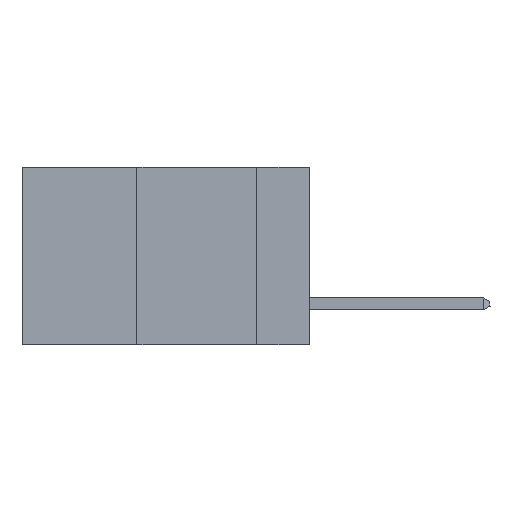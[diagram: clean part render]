
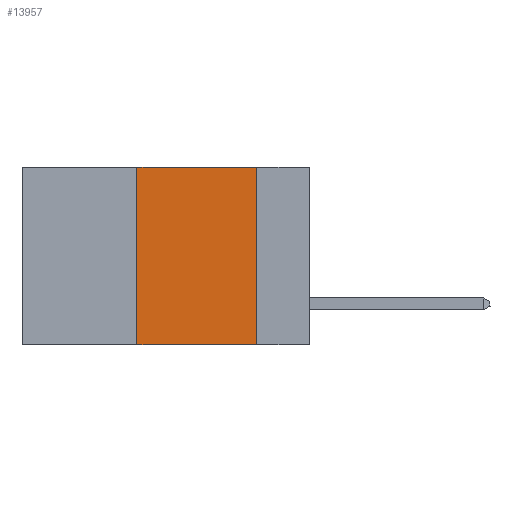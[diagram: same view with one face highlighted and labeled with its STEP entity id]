
A CAD part, left-side view. The second image highlights one B-rep face of the part: STEP entity #13957.
In plain terms, the highlighted planar face has unit normal (-1, 0, 0).
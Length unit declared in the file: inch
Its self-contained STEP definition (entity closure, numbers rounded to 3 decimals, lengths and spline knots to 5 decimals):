
#29 = CARTESIAN_POINT ( 'NONE',  ( 0., 0.6, 0. ) ) ;
#192 = EDGE_CURVE ( 'NONE', #10372, #8688, #6250, .T. ) ;
#811 = CARTESIAN_POINT ( 'NONE',  ( 0., 0.11, 0. ) ) ;
#1330 = DIRECTION ( 'NONE',  ( 0., -1., 0. ) ) ;
#1758 = DIRECTION ( 'NONE',  ( 0., 0., -1. ) ) ;
#2094 = VERTEX_POINT ( 'NONE', #15058 ) ;
#2177 = VECTOR ( 'NONE', #12289, 39.37008 ) ;
#3598 = EDGE_CURVE ( 'NONE', #16741, #2094, #14230, .T. ) ;
#3668 = ORIENTED_EDGE ( 'NONE', *, *, #14912, .F. ) ;
#4338 = CARTESIAN_POINT ( 'NONE',  ( 0., 0.36, 0. ) ) ;
#4455 = LINE ( 'NONE', #6945, #8726 ) ;
#4840 = ORIENTED_EDGE ( 'NONE', *, *, #192, .F. ) ;
#5137 = LINE ( 'NONE', #811, #6382 ) ;
#5692 = CARTESIAN_POINT ( 'NONE',  ( 0., 0.6, -0.37 ) ) ;
#6250 = LINE ( 'NONE', #29, #16333 ) ;
#6382 = VECTOR ( 'NONE', #13944, 39.37008 ) ;
#6945 = CARTESIAN_POINT ( 'NONE',  ( 0., 0.36, 0. ) ) ;
#8084 = DIRECTION ( 'NONE',  ( 0., 0., 1. ) ) ;
#8536 = EDGE_LOOP ( 'NONE', ( #3668, #4840, #15278, #11875 ) ) ;
#8688 = VERTEX_POINT ( 'NONE', #14435 ) ;
#8726 = VECTOR ( 'NONE', #8084, 39.37008 ) ;
#9553 = FACE_OUTER_BOUND ( 'NONE', #8536, .T. ) ;
#10372 = VERTEX_POINT ( 'NONE', #4338 ) ;
#11875 = ORIENTED_EDGE ( 'NONE', *, *, #3598, .T. ) ;
#12289 = DIRECTION ( 'NONE',  ( 0., -1., 0. ) ) ;
#13046 = AXIS2_PLACEMENT_3D ( 'NONE', #14972, #13509, #1758 ) ;
#13509 = DIRECTION ( 'NONE',  ( 1., 0., 0. ) ) ;
#13944 = DIRECTION ( 'NONE',  ( 0., 0., -1. ) ) ;
#13957 = ADVANCED_FACE ( 'NONE', ( #9553 ), #14910, .F. ) ;
#14230 = LINE ( 'NONE', #5692, #2177 ) ;
#14435 = CARTESIAN_POINT ( 'NONE',  ( 0., 0.11, 0. ) ) ;
#14504 = EDGE_CURVE ( 'NONE', #16741, #10372, #4455, .T. ) ;
#14910 = PLANE ( 'NONE',  #13046 ) ;
#14912 = EDGE_CURVE ( 'NONE', #8688, #2094, #5137, .T. ) ;
#14972 = CARTESIAN_POINT ( 'NONE',  ( 0., 0.6, 0. ) ) ;
#15058 = CARTESIAN_POINT ( 'NONE',  ( 0., 0.11, -0.37 ) ) ;
#15213 = CARTESIAN_POINT ( 'NONE',  ( 0., 0.36, -0.37 ) ) ;
#15278 = ORIENTED_EDGE ( 'NONE', *, *, #14504, .F. ) ;
#16333 = VECTOR ( 'NONE', #1330, 39.37008 ) ;
#16741 = VERTEX_POINT ( 'NONE', #15213 ) ;
